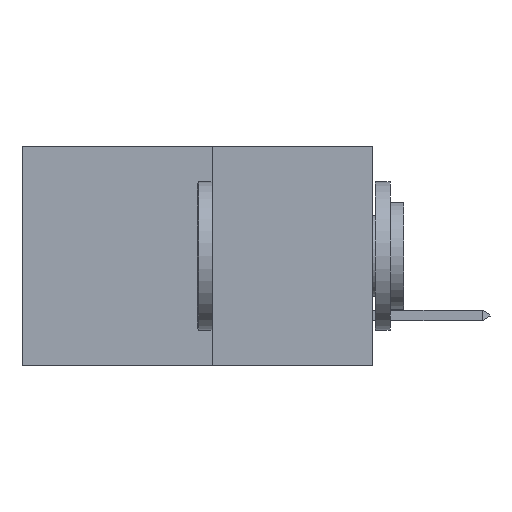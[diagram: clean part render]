
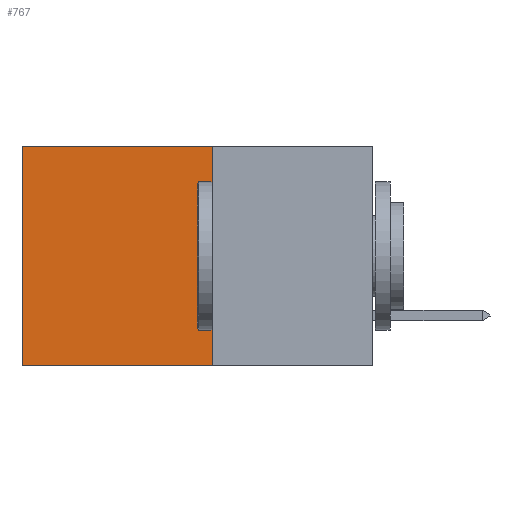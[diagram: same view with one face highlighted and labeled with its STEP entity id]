
A CAD part, left-side view. The second image highlights one B-rep face of the part: STEP entity #767.
In plain terms, the highlighted planar face has unit normal (-1, 0, 0).
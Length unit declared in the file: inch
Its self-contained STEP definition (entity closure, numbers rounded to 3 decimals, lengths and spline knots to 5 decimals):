
#767 = ADVANCED_FACE ( 'NONE', ( #2926 ), #7040, .F. ) ;
#1139 = DIRECTION ( 'NONE',  ( 0., 0., -1. ) ) ;
#2173 = ORIENTED_EDGE ( 'NONE', *, *, #11730, .T. ) ;
#2454 = VERTEX_POINT ( 'NONE', #6634 ) ;
#2674 = EDGE_CURVE ( 'NONE', #2985, #2454, #4544, .T. ) ;
#2926 = FACE_OUTER_BOUND ( 'NONE', #9327, .T. ) ;
#2985 = VERTEX_POINT ( 'NONE', #11786 ) ;
#3235 = ORIENTED_EDGE ( 'NONE', *, *, #4505, .T. ) ;
#3479 = VECTOR ( 'NONE', #10127, 39.37008 ) ;
#3508 = CARTESIAN_POINT ( 'NONE',  ( 0.277, 0.27, -0.37 ) ) ;
#4443 = VECTOR ( 'NONE', #4590, 39.37008 ) ;
#4449 = CARTESIAN_POINT ( 'NONE',  ( 0.277, 0.59, 0. ) ) ;
#4505 = EDGE_CURVE ( 'NONE', #10235, #12600, #9229, .T. ) ;
#4544 = LINE ( 'NONE', #10378, #12861 ) ;
#4590 = DIRECTION ( 'NONE',  ( 0., 1., 0. ) ) ;
#5474 = ORIENTED_EDGE ( 'NONE', *, *, #10288, .F. ) ;
#6634 = CARTESIAN_POINT ( 'NONE',  ( 0.277, 0.27, -0.37 ) ) ;
#7040 = PLANE ( 'NONE',  #13582 ) ;
#7060 = DIRECTION ( 'NONE',  ( 0., 0., -1. ) ) ;
#7082 = DIRECTION ( 'NONE',  ( 1., 0., 0. ) ) ;
#7531 = ORIENTED_EDGE ( 'NONE', *, *, #2674, .F. ) ;
#7755 = LINE ( 'NONE', #9030, #10374 ) ;
#9030 = CARTESIAN_POINT ( 'NONE',  ( 0.277, 0.27, 0. ) ) ;
#9229 = LINE ( 'NONE', #13906, #3479 ) ;
#9327 = EDGE_LOOP ( 'NONE', ( #3235, #5474, #7531, #2173 ) ) ;
#10127 = DIRECTION ( 'NONE',  ( 0., 0., -1. ) ) ;
#10235 = VERTEX_POINT ( 'NONE', #4449 ) ;
#10288 = EDGE_CURVE ( 'NONE', #2454, #12600, #13080, .T. ) ;
#10374 = VECTOR ( 'NONE', #13335, 39.37008 ) ;
#10378 = CARTESIAN_POINT ( 'NONE',  ( 0.277, 0.27, -0.37 ) ) ;
#10556 = CARTESIAN_POINT ( 'NONE',  ( 0.277, 0.59, -0.37 ) ) ;
#11730 = EDGE_CURVE ( 'NONE', #2985, #10235, #7755, .T. ) ;
#11786 = CARTESIAN_POINT ( 'NONE',  ( 0.277, 0.27, 0. ) ) ;
#12600 = VERTEX_POINT ( 'NONE', #10556 ) ;
#12614 = CARTESIAN_POINT ( 'NONE',  ( 0.277, 0.27, -0.37 ) ) ;
#12861 = VECTOR ( 'NONE', #1139, 39.37008 ) ;
#13080 = LINE ( 'NONE', #3508, #4443 ) ;
#13335 = DIRECTION ( 'NONE',  ( 0., 1., 0. ) ) ;
#13582 = AXIS2_PLACEMENT_3D ( 'NONE', #12614, #7082, #7060 ) ;
#13906 = CARTESIAN_POINT ( 'NONE',  ( 0.277, 0.59, -0.37 ) ) ;
